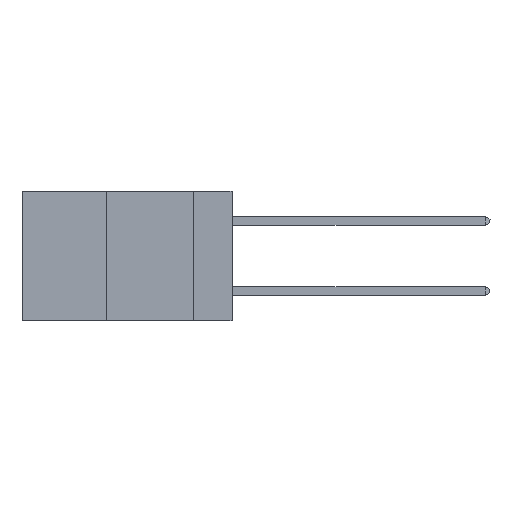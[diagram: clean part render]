
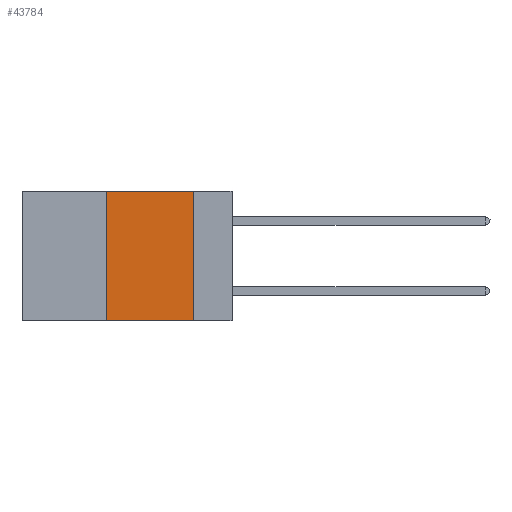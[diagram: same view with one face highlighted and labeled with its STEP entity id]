
A CAD part, left-side view. The second image highlights one B-rep face of the part: STEP entity #43784.
In plain terms, the highlighted planar face has unit normal (-1, 0, 0).
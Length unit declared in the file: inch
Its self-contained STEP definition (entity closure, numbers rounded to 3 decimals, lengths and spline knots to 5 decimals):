
#12 = VERTEX_POINT ( 'NONE', #25886 ) ;
#39 = CARTESIAN_POINT ( 'NONE',  ( 0., 0.6, 0. ) ) ;
#1847 = VECTOR ( 'NONE', #5558, 39.37008 ) ;
#2471 = DIRECTION ( 'NONE',  ( 1., 0., 0. ) ) ;
#3119 = VERTEX_POINT ( 'NONE', #27102 ) ;
#3164 = EDGE_LOOP ( 'NONE', ( #44679, #22600, #42302, #44468 ) ) ;
#3789 = EDGE_CURVE ( 'NONE', #3119, #17355, #19571, .T. ) ;
#5067 = VECTOR ( 'NONE', #45435, 39.37008 ) ;
#5558 = DIRECTION ( 'NONE',  ( 0., 0., 1. ) ) ;
#6391 = CARTESIAN_POINT ( 'NONE',  ( 0., 0.6, -0.37 ) ) ;
#10403 = VECTOR ( 'NONE', #42400, 39.37008 ) ;
#13491 = LINE ( 'NONE', #6391, #30028 ) ;
#13527 = DIRECTION ( 'NONE',  ( 0., -1., 0. ) ) ;
#14384 = AXIS2_PLACEMENT_3D ( 'NONE', #37751, #2471, #27234 ) ;
#15619 = LINE ( 'NONE', #41888, #5067 ) ;
#17355 = VERTEX_POINT ( 'NONE', #34910 ) ;
#19571 = LINE ( 'NONE', #37395, #1847 ) ;
#20395 = EDGE_CURVE ( 'NONE', #12, #21583, #15619, .T. ) ;
#21583 = VERTEX_POINT ( 'NONE', #41799 ) ;
#22600 = ORIENTED_EDGE ( 'NONE', *, *, #35078, .F. ) ;
#23682 = PLANE ( 'NONE',  #14384 ) ;
#24140 = EDGE_CURVE ( 'NONE', #3119, #21583, #13491, .T. ) ;
#25886 = CARTESIAN_POINT ( 'NONE',  ( 0., 0.11, 0. ) ) ;
#27102 = CARTESIAN_POINT ( 'NONE',  ( 0., 0.36, -0.37 ) ) ;
#27234 = DIRECTION ( 'NONE',  ( 0., 0., -1. ) ) ;
#30028 = VECTOR ( 'NONE', #13527, 39.37008 ) ;
#30278 = LINE ( 'NONE', #39, #10403 ) ;
#34910 = CARTESIAN_POINT ( 'NONE',  ( 0., 0.36, 0. ) ) ;
#35078 = EDGE_CURVE ( 'NONE', #17355, #12, #30278, .T. ) ;
#36823 = FACE_OUTER_BOUND ( 'NONE', #3164, .T. ) ;
#37395 = CARTESIAN_POINT ( 'NONE',  ( 0., 0.36, 0. ) ) ;
#37751 = CARTESIAN_POINT ( 'NONE',  ( 0., 0.6, 0. ) ) ;
#41799 = CARTESIAN_POINT ( 'NONE',  ( 0., 0.11, -0.37 ) ) ;
#41888 = CARTESIAN_POINT ( 'NONE',  ( 0., 0.11, 0. ) ) ;
#42302 = ORIENTED_EDGE ( 'NONE', *, *, #3789, .F. ) ;
#42400 = DIRECTION ( 'NONE',  ( 0., -1., 0. ) ) ;
#43784 = ADVANCED_FACE ( 'NONE', ( #36823 ), #23682, .F. ) ;
#44468 = ORIENTED_EDGE ( 'NONE', *, *, #24140, .T. ) ;
#44679 = ORIENTED_EDGE ( 'NONE', *, *, #20395, .F. ) ;
#45435 = DIRECTION ( 'NONE',  ( 0., 0., -1. ) ) ;
